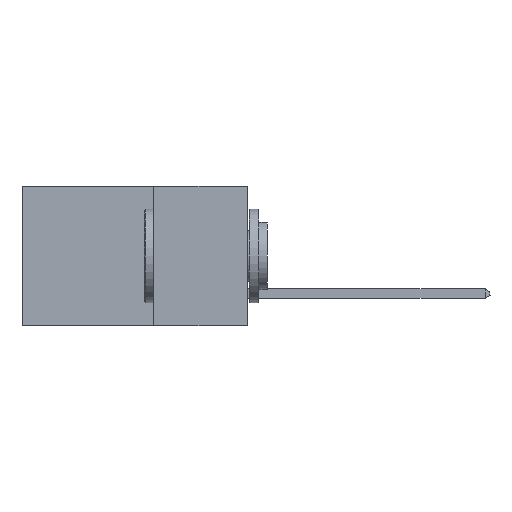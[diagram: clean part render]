
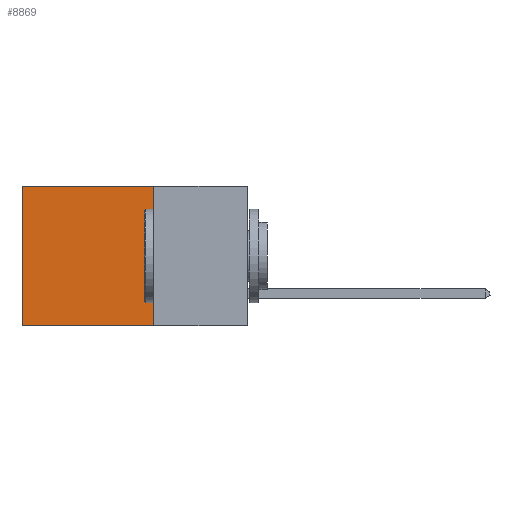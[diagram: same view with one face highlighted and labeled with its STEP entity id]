
A CAD part, left-side view. The second image highlights one B-rep face of the part: STEP entity #8869.
In plain terms, the highlighted planar face has unit normal (-1, 0, 0).
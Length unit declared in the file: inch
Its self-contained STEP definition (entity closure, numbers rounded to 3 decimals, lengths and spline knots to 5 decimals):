
#969 = EDGE_CURVE ( 'NONE', #14829, #6000, #2958, .T. ) ;
#1250 = DIRECTION ( 'NONE',  ( 0., 1., 0. ) ) ;
#2488 = ORIENTED_EDGE ( 'NONE', *, *, #5692, .T. ) ;
#2810 = ORIENTED_EDGE ( 'NONE', *, *, #7549, .F. ) ;
#2958 = LINE ( 'NONE', #12055, #3514 ) ;
#3164 = FACE_OUTER_BOUND ( 'NONE', #9263, .T. ) ;
#3201 = VECTOR ( 'NONE', #1250, 39.37008 ) ;
#3419 = ORIENTED_EDGE ( 'NONE', *, *, #6410, .T. ) ;
#3514 = VECTOR ( 'NONE', #13250, 39.37008 ) ;
#3981 = CARTESIAN_POINT ( 'NONE',  ( 0.298, 0.6, 0. ) ) ;
#4581 = DIRECTION ( 'NONE',  ( 0., 1., 0. ) ) ;
#5692 = EDGE_CURVE ( 'NONE', #14829, #11372, #15090, .T. ) ;
#5887 = CARTESIAN_POINT ( 'NONE',  ( 0.298, 0.25, 0. ) ) ;
#5948 = CARTESIAN_POINT ( 'NONE',  ( 0.298, 0.25, 0. ) ) ;
#6000 = VERTEX_POINT ( 'NONE', #8535 ) ;
#6410 = EDGE_CURVE ( 'NONE', #11372, #7330, #9893, .T. ) ;
#6959 = VECTOR ( 'NONE', #4581, 39.37008 ) ;
#7047 = DIRECTION ( 'NONE',  ( 1., 0., 0. ) ) ;
#7330 = VERTEX_POINT ( 'NONE', #9001 ) ;
#7549 = EDGE_CURVE ( 'NONE', #6000, #7330, #12086, .T. ) ;
#8326 = CARTESIAN_POINT ( 'NONE',  ( 0.298, 0.25, -0.37 ) ) ;
#8415 = VECTOR ( 'NONE', #13598, 39.37008 ) ;
#8535 = CARTESIAN_POINT ( 'NONE',  ( 0.298, 0.25, -0.37 ) ) ;
#8869 = ADVANCED_FACE ( 'NONE', ( #3164 ), #12966, .F. ) ;
#9001 = CARTESIAN_POINT ( 'NONE',  ( 0.298, 0.6, -0.37 ) ) ;
#9263 = EDGE_LOOP ( 'NONE', ( #3419, #2810, #15096, #2488 ) ) ;
#9648 = CARTESIAN_POINT ( 'NONE',  ( 0.298, 0.6, 0. ) ) ;
#9893 = LINE ( 'NONE', #9648, #8415 ) ;
#11372 = VERTEX_POINT ( 'NONE', #3981 ) ;
#11652 = CARTESIAN_POINT ( 'NONE',  ( 0.298, 0.25, 0. ) ) ;
#11710 = DIRECTION ( 'NONE',  ( 0., 0., -1. ) ) ;
#12055 = CARTESIAN_POINT ( 'NONE',  ( 0.298, 0.25, 0. ) ) ;
#12086 = LINE ( 'NONE', #8326, #3201 ) ;
#12571 = AXIS2_PLACEMENT_3D ( 'NONE', #5887, #7047, #11710 ) ;
#12966 = PLANE ( 'NONE',  #12571 ) ;
#13250 = DIRECTION ( 'NONE',  ( 0., 0., -1. ) ) ;
#13598 = DIRECTION ( 'NONE',  ( 0., 0., -1. ) ) ;
#14829 = VERTEX_POINT ( 'NONE', #5948 ) ;
#15090 = LINE ( 'NONE', #11652, #6959 ) ;
#15096 = ORIENTED_EDGE ( 'NONE', *, *, #969, .F. ) ;
